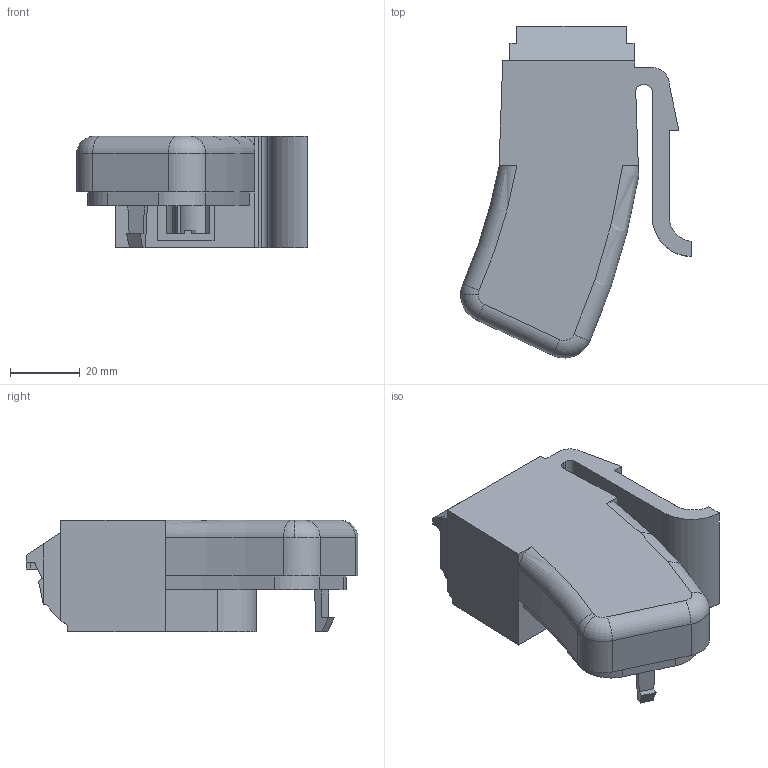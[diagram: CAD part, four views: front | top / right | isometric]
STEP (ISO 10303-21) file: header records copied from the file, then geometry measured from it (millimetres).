
FILE_DESCRIPTION (( 'STEP AP214' ), '1' );
FILE_NAME ('mag_right.STEP', '2013-09-24T00:09:23', ( '' ), ( '' ), 'SwSTEP 2.0', 'SolidWorks 2013', '' );
FILE_SCHEMA (( 'AUTOMOTIVE_DESIGN' ));
Length unit declared in the file: millimetre
Products named in the file (1): mag_right
Bounding box: 66.25 x 95.38 x 32 mm (x, y, z)
Volume: 61079.1 mm3; surface area: 26548.6 mm2
Topology: 1 solids, 1 shells, 168 faces, 481 edges, 314 vertices
Faces by surface type: plane 102, cylinder 53, torus 10, bspline 3
Entity records: 5678 total; most frequent: CARTESIAN_POINT 1218, ORIENTED_EDGE 962, DIRECTION 912, EDGE_CURVE 481, VECTOR 320, LINE 320, VERTEX_POINT 314, AXIS2_PLACEMENT_3D 296
